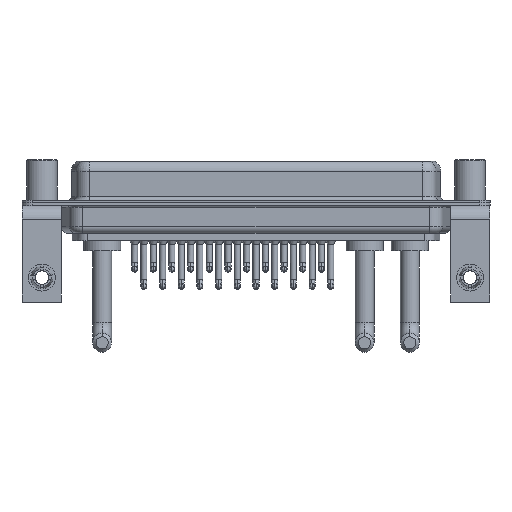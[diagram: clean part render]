
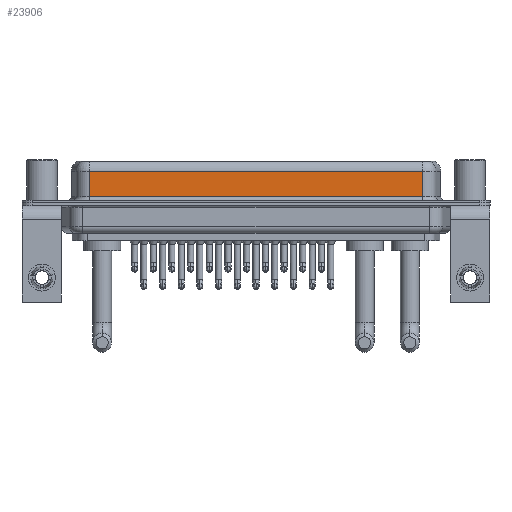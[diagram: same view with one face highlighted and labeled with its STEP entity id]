
A CAD part, front view. The second image highlights one B-rep face of the part: STEP entity #23906.
In plain terms, the highlighted planar face has unit normal (0, -1, 0).
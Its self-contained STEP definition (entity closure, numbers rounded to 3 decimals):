
#613 = AXIS2_PLACEMENT_3D ( 'NONE', #9909, #5357, #22389 ) ;
#1755 = CARTESIAN_POINT ( 'NONE',  ( 56.462, -3.95, 6.4 ) ) ;
#3070 = ORIENTED_EDGE ( 'NONE', *, *, #13414, .T. ) ;
#3539 = CARTESIAN_POINT ( 'NONE',  ( 56.462, -3.95, 0.9 ) ) ;
#5357 = DIRECTION ( 'NONE',  ( 0., 1., 0. ) ) ;
#6352 = VERTEX_POINT ( 'NONE', #25658 ) ;
#6998 = LINE ( 'NONE', #16384, #7481 ) ;
#7481 = VECTOR ( 'NONE', #20399, 1000. ) ;
#9624 = VECTOR ( 'NONE', #12387, 1000. ) ;
#9909 = CARTESIAN_POINT ( 'NONE',  ( 56.462, -3.95, 6.4 ) ) ;
#10229 = ORIENTED_EDGE ( 'NONE', *, *, #23504, .T. ) ;
#10497 = EDGE_CURVE ( 'NONE', #12193, #16160, #20694, .T. ) ;
#11688 = VECTOR ( 'NONE', #20826, 1000. ) ;
#12193 = VERTEX_POINT ( 'NONE', #14435 ) ;
#12303 = CARTESIAN_POINT ( 'NONE',  ( 7.038, -3.95, 4.65 ) ) ;
#12387 = DIRECTION ( 'NONE',  ( 0., 0., -1. ) ) ;
#12702 = EDGE_LOOP ( 'NONE', ( #26550, #3070, #15452, #10229 ) ) ;
#13414 = EDGE_CURVE ( 'NONE', #12193, #27211, #6998, .T. ) ;
#14435 = CARTESIAN_POINT ( 'NONE',  ( 56.462, -3.95, 4.65 ) ) ;
#15452 = ORIENTED_EDGE ( 'NONE', *, *, #26378, .T. ) ;
#15785 = CARTESIAN_POINT ( 'NONE',  ( 56.462, -3.95, 0.9 ) ) ;
#15974 = LINE ( 'NONE', #3539, #23122 ) ;
#16160 = VERTEX_POINT ( 'NONE', #15785 ) ;
#16260 = LINE ( 'NONE', #25133, #11688 ) ;
#16384 = CARTESIAN_POINT ( 'NONE',  ( 56.462, -3.95, 4.65 ) ) ;
#20399 = DIRECTION ( 'NONE',  ( -1., 0., 0. ) ) ;
#20694 = LINE ( 'NONE', #1755, #9624 ) ;
#20826 = DIRECTION ( 'NONE',  ( 0., 0., -1. ) ) ;
#22389 = DIRECTION ( 'NONE',  ( 0., 0., 1. ) ) ;
#23122 = VECTOR ( 'NONE', #24423, 1000. ) ;
#23504 = EDGE_CURVE ( 'NONE', #6352, #16160, #15974, .T. ) ;
#23906 = ADVANCED_FACE ( 'NONE', ( #26532 ), #24191, .F. ) ;
#24191 = PLANE ( 'NONE',  #613 ) ;
#24423 = DIRECTION ( 'NONE',  ( 1., 0., 0. ) ) ;
#25133 = CARTESIAN_POINT ( 'NONE',  ( 7.038, -3.95, 6.4 ) ) ;
#25658 = CARTESIAN_POINT ( 'NONE',  ( 7.038, -3.95, 0.9 ) ) ;
#26378 = EDGE_CURVE ( 'NONE', #27211, #6352, #16260, .T. ) ;
#26532 = FACE_OUTER_BOUND ( 'NONE', #12702, .T. ) ;
#26550 = ORIENTED_EDGE ( 'NONE', *, *, #10497, .F. ) ;
#27211 = VERTEX_POINT ( 'NONE', #12303 ) ;
